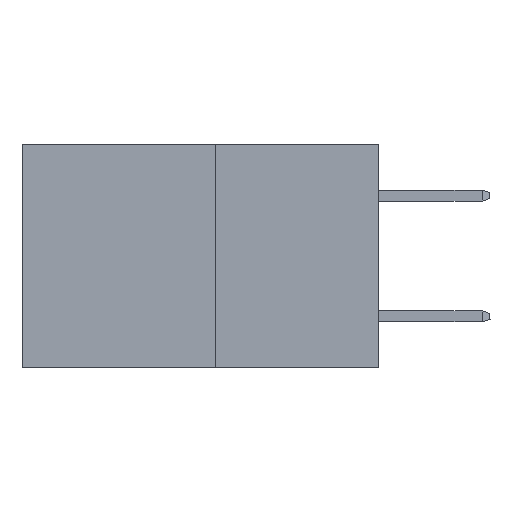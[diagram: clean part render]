
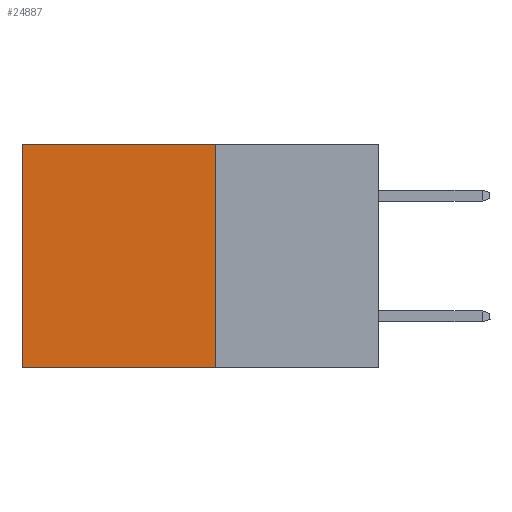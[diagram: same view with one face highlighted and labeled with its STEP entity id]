
A CAD part, left-side view. The second image highlights one B-rep face of the part: STEP entity #24887.
In plain terms, the highlighted planar face has unit normal (-1, 0, 0).
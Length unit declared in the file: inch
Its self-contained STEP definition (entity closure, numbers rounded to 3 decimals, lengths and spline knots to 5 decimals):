
#354 = ORIENTED_EDGE ( 'NONE', *, *, #15259, .F. ) ;
#1008 = EDGE_LOOP ( 'NONE', ( #23743, #354, #23141, #18674 ) ) ;
#2722 = CARTESIAN_POINT ( 'NONE',  ( 0.277, 0.59, -0.37 ) ) ;
#3563 = DIRECTION ( 'NONE',  ( 0., 1., 0. ) ) ;
#4882 = CARTESIAN_POINT ( 'NONE',  ( 0.277, 0.27, 0. ) ) ;
#5544 = AXIS2_PLACEMENT_3D ( 'NONE', #12076, #26214, #14126 ) ;
#5550 = CARTESIAN_POINT ( 'NONE',  ( 0.277, 0.27, -0.37 ) ) ;
#5689 = CARTESIAN_POINT ( 'NONE',  ( 0.277, 0.59, -0.37 ) ) ;
#6883 = CARTESIAN_POINT ( 'NONE',  ( 0.277, 0.59, 0. ) ) ;
#7632 = LINE ( 'NONE', #5689, #13080 ) ;
#8543 = LINE ( 'NONE', #15939, #13959 ) ;
#10384 = VERTEX_POINT ( 'NONE', #2722 ) ;
#11537 = VECTOR ( 'NONE', #11775, 39.37008 ) ;
#11775 = DIRECTION ( 'NONE',  ( 0., 1., 0. ) ) ;
#11842 = LINE ( 'NONE', #20481, #17298 ) ;
#11991 = EDGE_CURVE ( 'NONE', #18483, #10384, #7632, .T. ) ;
#12076 = CARTESIAN_POINT ( 'NONE',  ( 0.277, 0.27, -0.37 ) ) ;
#13080 = VECTOR ( 'NONE', #20021, 39.37008 ) ;
#13959 = VECTOR ( 'NONE', #3563, 39.37008 ) ;
#14126 = DIRECTION ( 'NONE',  ( 0., 0., -1. ) ) ;
#14973 = VERTEX_POINT ( 'NONE', #21203 ) ;
#15259 = EDGE_CURVE ( 'NONE', #14973, #10384, #17001, .T. ) ;
#15505 = EDGE_CURVE ( 'NONE', #22995, #14973, #11842, .T. ) ;
#15939 = CARTESIAN_POINT ( 'NONE',  ( 0.277, 0.27, 0. ) ) ;
#16162 = FACE_OUTER_BOUND ( 'NONE', #1008, .T. ) ;
#16434 = DIRECTION ( 'NONE',  ( 0., 0., -1. ) ) ;
#17001 = LINE ( 'NONE', #5550, #11537 ) ;
#17298 = VECTOR ( 'NONE', #16434, 39.37008 ) ;
#17383 = EDGE_CURVE ( 'NONE', #22995, #18483, #8543, .T. ) ;
#18483 = VERTEX_POINT ( 'NONE', #6883 ) ;
#18674 = ORIENTED_EDGE ( 'NONE', *, *, #17383, .T. ) ;
#20021 = DIRECTION ( 'NONE',  ( 0., 0., -1. ) ) ;
#20481 = CARTESIAN_POINT ( 'NONE',  ( 0.277, 0.27, -0.37 ) ) ;
#21203 = CARTESIAN_POINT ( 'NONE',  ( 0.277, 0.27, -0.37 ) ) ;
#22995 = VERTEX_POINT ( 'NONE', #4882 ) ;
#23141 = ORIENTED_EDGE ( 'NONE', *, *, #15505, .F. ) ;
#23743 = ORIENTED_EDGE ( 'NONE', *, *, #11991, .T. ) ;
#24205 = PLANE ( 'NONE',  #5544 ) ;
#24887 = ADVANCED_FACE ( 'NONE', ( #16162 ), #24205, .F. ) ;
#26214 = DIRECTION ( 'NONE',  ( 1., 0., 0. ) ) ;
